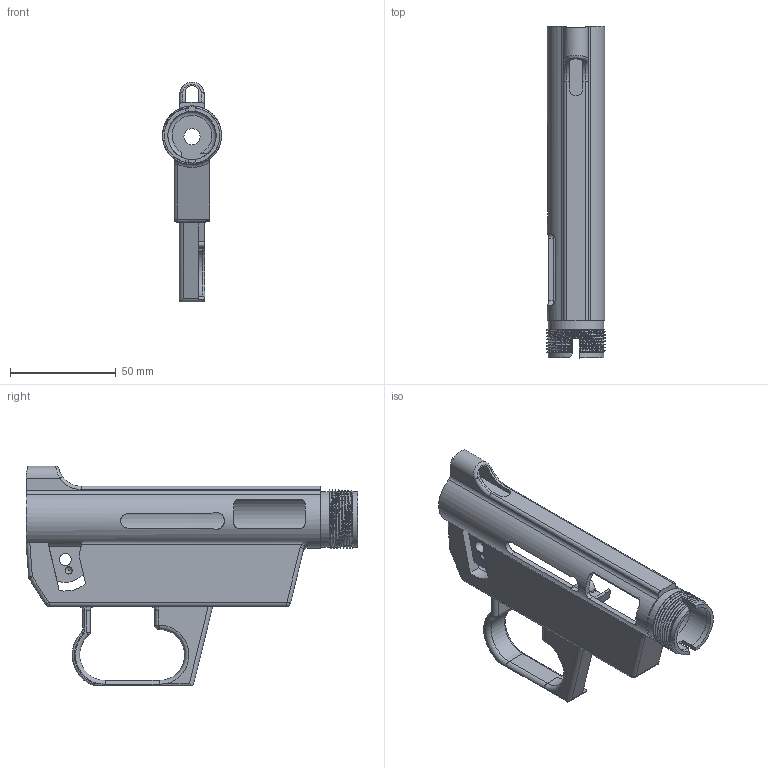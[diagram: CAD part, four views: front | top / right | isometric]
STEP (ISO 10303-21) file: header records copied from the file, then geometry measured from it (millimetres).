
FILE_DESCRIPTION(/* description */ (''),/* implementation_level */ '2;1');
FILE_NAME(/* name */ 'AR-7 Raw Measurements - NOT FOR PRINTING.step',/* time_stamp */ '2020-12-07T22:02:56-05:00',/* author */ (''),/* organization */ (''),/* preprocessor_version */ 'ST-DEVELOPER v18.1',/* originating_system */ 'Autodesk Translation Framework v9.3.0.1241',/* authorisation */ '');
FILE_SCHEMA (('AUTOMOTIVE_DESIGN { 1 0 10303 214 3 1 1 }'));
Length unit declared in the file: millimetre
Products named in the file (1): Reciever
Bounding box: 27.85 x 156.95 x 103.93 mm (x, y, z)
Volume: 51985.6 mm3; surface area: 40678.2 mm2
Topology: 4 solids, 4 shells, 304 faces, 849 edges, 551 vertices
Faces by surface type: plane 134, cylinder 122, bspline 32, torus 14, sphere 2
Full cylindrical faces by diameter (mm): 3.45 x1, 3.75 x1, 3.95 x2, 5.22 x1, 5.65 x1, 5.8 x1, 7.65 x1, 7.75 x1, 22.9 x2, 26.132 x2, 26.3 x1, 27.85 x3
Entity records: 12642 total; most frequent: CARTESIAN_POINT 4919, ORIENTED_EDGE 1696, DIRECTION 1506, EDGE_CURVE 848, VERTEX_POINT 551, AXIS2_PLACEMENT_3D 524, LINE 458, VECTOR 458
